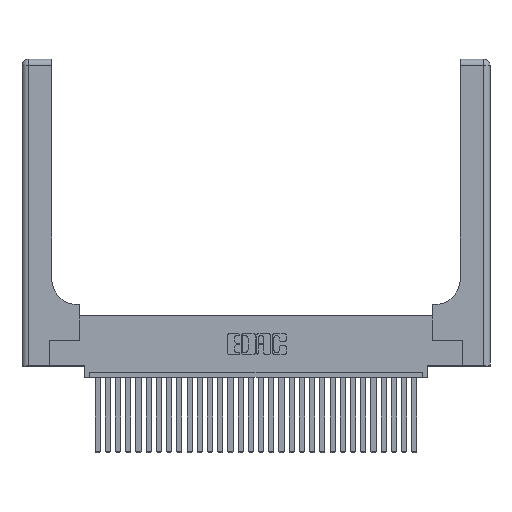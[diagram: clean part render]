
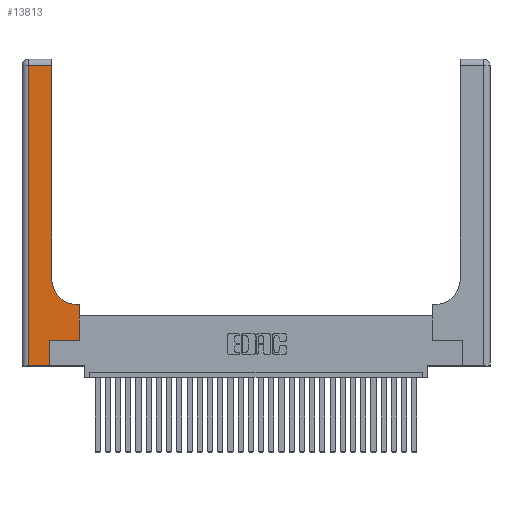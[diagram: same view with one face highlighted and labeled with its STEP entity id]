
A CAD part, top view. The second image highlights one B-rep face of the part: STEP entity #13813.
In plain terms, the highlighted planar face has unit normal (0, 0, 1).
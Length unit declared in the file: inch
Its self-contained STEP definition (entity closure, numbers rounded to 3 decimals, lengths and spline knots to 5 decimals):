
#45 = DIRECTION ( 'NONE',  ( 0., 1., 0. ) ) ;
#235 = ORIENTED_EDGE ( 'NONE', *, *, #2412, .T. ) ;
#1560 = CARTESIAN_POINT ( 'NONE',  ( 0.2915, 0.6, 0.37 ) ) ;
#1819 = CARTESIAN_POINT ( 'NONE',  ( 0.06, 3., 0.37 ) ) ;
#2412 = EDGE_CURVE ( 'NONE', #29445, #28065, #21885, .T. ) ;
#2425 = LINE ( 'NONE', #3274, #17629 ) ;
#2600 = ORIENTED_EDGE ( 'NONE', *, *, #19499, .T. ) ;
#2761 = CARTESIAN_POINT ( 'NONE',  ( 0.269, 0.25, 0.37 ) ) ;
#3274 = CARTESIAN_POINT ( 'NONE',  ( 0., 2.94, 0.37 ) ) ;
#3332 = VECTOR ( 'NONE', #45, 39.37008 ) ;
#4821 = CARTESIAN_POINT ( 'NONE',  ( 0.269, 0., 0.37 ) ) ;
#4876 = DIRECTION ( 'NONE',  ( 1., 0., 0. ) ) ;
#4966 = EDGE_LOOP ( 'NONE', ( #235, #17827, #2600, #11704, #29610, #12321, #29778, #6904, #26586 ) ) ;
#5099 = VERTEX_POINT ( 'NONE', #5714 ) ;
#5162 = CARTESIAN_POINT ( 'NONE',  ( 0.5585, 0.6, 0.37 ) ) ;
#5699 = VECTOR ( 'NONE', #18126, 39.37008 ) ;
#5714 = CARTESIAN_POINT ( 'NONE',  ( 0.06, 0., 0.37 ) ) ;
#5871 = VERTEX_POINT ( 'NONE', #20442 ) ;
#6396 = VERTEX_POINT ( 'NONE', #15773 ) ;
#6904 = ORIENTED_EDGE ( 'NONE', *, *, #15337, .T. ) ;
#7573 = VECTOR ( 'NONE', #13496, 39.37008 ) ;
#8155 = CARTESIAN_POINT ( 'NONE',  ( 0.5585, 0.25, 0.37 ) ) ;
#9317 = CARTESIAN_POINT ( 'NONE',  ( 0.5585, 0.25, 0.37 ) ) ;
#9323 = CARTESIAN_POINT ( 'NONE',  ( 0.2915, 2.94, 0.37 ) ) ;
#10465 = EDGE_CURVE ( 'NONE', #28065, #5871, #2425, .T. ) ;
#10731 = CARTESIAN_POINT ( 'NONE',  ( 0., 0., 0.37 ) ) ;
#11634 = DIRECTION ( 'NONE',  ( 0., 1., 0. ) ) ;
#11704 = ORIENTED_EDGE ( 'NONE', *, *, #20218, .T. ) ;
#12001 = EDGE_CURVE ( 'NONE', #23026, #29445, #28000, .T. ) ;
#12321 = ORIENTED_EDGE ( 'NONE', *, *, #29427, .T. ) ;
#12504 = PLANE ( 'NONE',  #20753 ) ;
#12707 = CARTESIAN_POINT ( 'NONE',  ( 0., 3., 0.37 ) ) ;
#13496 = DIRECTION ( 'NONE',  ( 0., -1., 0. ) ) ;
#13813 = ADVANCED_FACE ( 'NONE', ( #21273 ), #12504, .F. ) ;
#14200 = CARTESIAN_POINT ( 'NONE',  ( 0.5415, 0.6, 0.37 ) ) ;
#14702 = DIRECTION ( 'NONE',  ( 0., 0., -1. ) ) ;
#14975 = LINE ( 'NONE', #2761, #22683 ) ;
#15229 = AXIS2_PLACEMENT_3D ( 'NONE', #21713, #14702, #4876 ) ;
#15286 = DIRECTION ( 'NONE',  ( -1., 0., 0. ) ) ;
#15337 = EDGE_CURVE ( 'NONE', #28716, #23026, #26368, .T. ) ;
#15773 = CARTESIAN_POINT ( 'NONE',  ( 0.269, 0.25, 0.37 ) ) ;
#15915 = LINE ( 'NONE', #9317, #3332 ) ;
#16352 = VECTOR ( 'NONE', #11634, 39.37008 ) ;
#16551 = VERTEX_POINT ( 'NONE', #8155 ) ;
#17629 = VECTOR ( 'NONE', #15286, 39.37008 ) ;
#17697 = VECTOR ( 'NONE', #22286, 39.37008 ) ;
#17827 = ORIENTED_EDGE ( 'NONE', *, *, #10465, .T. ) ;
#18126 = DIRECTION ( 'NONE',  ( -1., 0., 0. ) ) ;
#18675 = LINE ( 'NONE', #1819, #7573 ) ;
#18874 = VERTEX_POINT ( 'NONE', #4821 ) ;
#19009 = LINE ( 'NONE', #10731, #24151 ) ;
#19499 = EDGE_CURVE ( 'NONE', #5871, #5099, #18675, .T. ) ;
#19516 = CARTESIAN_POINT ( 'NONE',  ( 0.2915, 0.85, 0.37 ) ) ;
#20218 = EDGE_CURVE ( 'NONE', #5099, #18874, #19009, .T. ) ;
#20442 = CARTESIAN_POINT ( 'NONE',  ( 0.06, 2.94, 0.37 ) ) ;
#20753 = AXIS2_PLACEMENT_3D ( 'NONE', #12707, #21919, #22310 ) ;
#21273 = FACE_OUTER_BOUND ( 'NONE', #4966, .T. ) ;
#21713 = CARTESIAN_POINT ( 'NONE',  ( 0.5415, 0.85, 0.37 ) ) ;
#21885 = LINE ( 'NONE', #28481, #16352 ) ;
#21919 = DIRECTION ( 'NONE',  ( 0., 0., -1. ) ) ;
#22286 = DIRECTION ( 'NONE',  ( 0., 1., 0. ) ) ;
#22310 = DIRECTION ( 'NONE',  ( -1., 0., 0. ) ) ;
#22619 = DIRECTION ( 'NONE',  ( 1., 0., 0. ) ) ;
#22683 = VECTOR ( 'NONE', #28568, 39.37008 ) ;
#23026 = VERTEX_POINT ( 'NONE', #14200 ) ;
#23159 = LINE ( 'NONE', #24123, #17697 ) ;
#24123 = CARTESIAN_POINT ( 'NONE',  ( 0.269, 0., 0.37 ) ) ;
#24151 = VECTOR ( 'NONE', #22619, 39.37008 ) ;
#26368 = LINE ( 'NONE', #1560, #5699 ) ;
#26511 = EDGE_CURVE ( 'NONE', #16551, #28716, #15915, .T. ) ;
#26586 = ORIENTED_EDGE ( 'NONE', *, *, #12001, .T. ) ;
#27719 = EDGE_CURVE ( 'NONE', #18874, #6396, #23159, .T. ) ;
#28000 = CIRCLE ( 'NONE', #15229, 0.25 ) ;
#28065 = VERTEX_POINT ( 'NONE', #9323 ) ;
#28481 = CARTESIAN_POINT ( 'NONE',  ( 0.2915, 3., 0.37 ) ) ;
#28568 = DIRECTION ( 'NONE',  ( 1., 0., 0. ) ) ;
#28716 = VERTEX_POINT ( 'NONE', #5162 ) ;
#29427 = EDGE_CURVE ( 'NONE', #6396, #16551, #14975, .T. ) ;
#29445 = VERTEX_POINT ( 'NONE', #19516 ) ;
#29610 = ORIENTED_EDGE ( 'NONE', *, *, #27719, .T. ) ;
#29778 = ORIENTED_EDGE ( 'NONE', *, *, #26511, .T. ) ;
